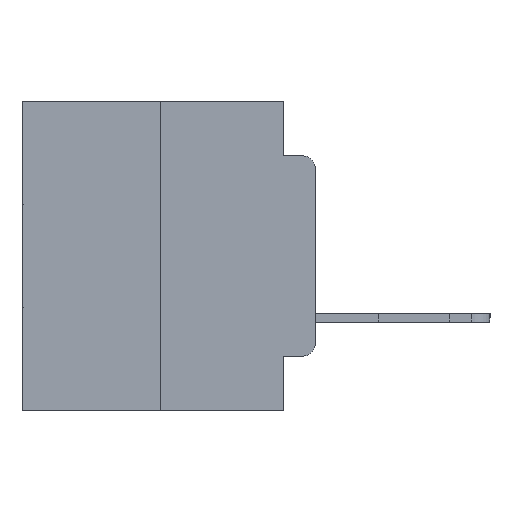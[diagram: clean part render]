
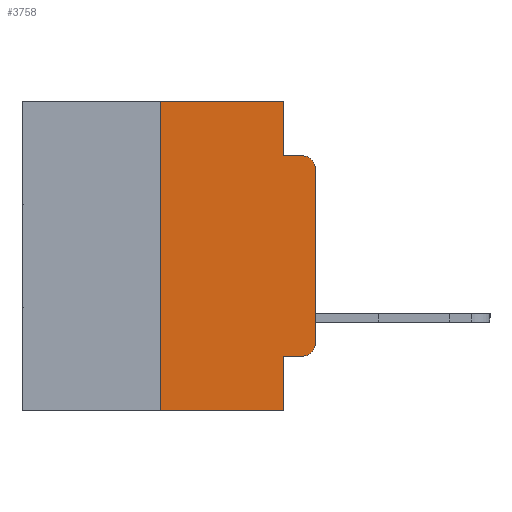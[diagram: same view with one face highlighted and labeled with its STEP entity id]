
A CAD part, left-side view. The second image highlights one B-rep face of the part: STEP entity #3758.
In plain terms, the highlighted planar face has unit normal (-1, 0, 0).
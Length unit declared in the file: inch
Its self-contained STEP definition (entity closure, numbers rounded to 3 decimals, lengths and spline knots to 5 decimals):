
#509 = VERTEX_POINT ( 'NONE', #731 ) ;
#619 = EDGE_CURVE ( 'NONE', #2781, #13525, #25787, .T. ) ;
#653 = ORIENTED_EDGE ( 'NONE', *, *, #619, .T. ) ;
#731 = CARTESIAN_POINT ( 'NONE',  ( 0., 0.25, -0.5 ) ) ;
#1536 = CARTESIAN_POINT ( 'NONE',  ( 0., 0.02, -0.4115 ) ) ;
#1886 = CARTESIAN_POINT ( 'NONE',  ( 0., 0.051, -0.0885 ) ) ;
#1912 = VECTOR ( 'NONE', #22514, 39.37008 ) ;
#2169 = ORIENTED_EDGE ( 'NONE', *, *, #4892, .T. ) ;
#2703 = EDGE_CURVE ( 'NONE', #5322, #26396, #15294, .T. ) ;
#2781 = VERTEX_POINT ( 'NONE', #17299 ) ;
#3119 = CARTESIAN_POINT ( 'NONE',  ( 0., 0.051, -0.5 ) ) ;
#3184 = CARTESIAN_POINT ( 'NONE',  ( 0., 0.25, 0. ) ) ;
#3740 = VERTEX_POINT ( 'NONE', #11287 ) ;
#3758 = ADVANCED_FACE ( 'NONE', ( #14607 ), #15090, .F. ) ;
#3760 = VECTOR ( 'NONE', #12633, 39.37008 ) ;
#4326 = ORIENTED_EDGE ( 'NONE', *, *, #18955, .F. ) ;
#4496 = DIRECTION ( 'NONE',  ( 0., -1., 0. ) ) ;
#4892 = EDGE_CURVE ( 'NONE', #13525, #3740, #17182, .T. ) ;
#5014 = ORIENTED_EDGE ( 'NONE', *, *, #11476, .T. ) ;
#5322 = VERTEX_POINT ( 'NONE', #23242 ) ;
#5421 = DIRECTION ( 'NONE',  ( 0., 0., 1. ) ) ;
#5715 = VERTEX_POINT ( 'NONE', #3119 ) ;
#7030 = ORIENTED_EDGE ( 'NONE', *, *, #26593, .T. ) ;
#7948 = CARTESIAN_POINT ( 'NONE',  ( 0., 0.473, 0. ) ) ;
#8159 = DIRECTION ( 'NONE',  ( 0., 0., -1. ) ) ;
#8310 = DIRECTION ( 'NONE',  ( 1., 0., 0. ) ) ;
#8346 = EDGE_LOOP ( 'NONE', ( #653, #2169, #19217, #15012, #25735, #4326, #5014, #10703, #22994, #7030 ) ) ;
#8348 = VERTEX_POINT ( 'NONE', #19682 ) ;
#8958 = DIRECTION ( 'NONE',  ( 0., 0., 1. ) ) ;
#9043 = DIRECTION ( 'NONE',  ( 0., -1., 0. ) ) ;
#9094 = CARTESIAN_POINT ( 'NONE',  ( 0., 0.02, -0.3915 ) ) ;
#9879 = CARTESIAN_POINT ( 'NONE',  ( 0., 0.02, -0.1085 ) ) ;
#10219 = VECTOR ( 'NONE', #9043, 39.37008 ) ;
#10496 = CARTESIAN_POINT ( 'NONE',  ( 0., 0.051, 0. ) ) ;
#10703 = ORIENTED_EDGE ( 'NONE', *, *, #16935, .F. ) ;
#11239 = DIRECTION ( 'NONE',  ( 0., 0., -1. ) ) ;
#11287 = CARTESIAN_POINT ( 'NONE',  ( 0., 0.02, -0.0885 ) ) ;
#11476 = EDGE_CURVE ( 'NONE', #509, #5715, #15886, .T. ) ;
#11786 = VECTOR ( 'NONE', #4496, 39.37008 ) ;
#11884 = CARTESIAN_POINT ( 'NONE',  ( 0., 0.051, 0. ) ) ;
#12022 = DIRECTION ( 'NONE',  ( 0., 0., -1. ) ) ;
#12633 = DIRECTION ( 'NONE',  ( 0., 0., -1. ) ) ;
#13525 = VERTEX_POINT ( 'NONE', #19213 ) ;
#14157 = LINE ( 'NONE', #14250, #23730 ) ;
#14250 = CARTESIAN_POINT ( 'NONE',  ( 0., 0.051, -0.4115 ) ) ;
#14607 = FACE_OUTER_BOUND ( 'NONE', #8346, .T. ) ;
#15012 = ORIENTED_EDGE ( 'NONE', *, *, #2703, .F. ) ;
#15090 = PLANE ( 'NONE',  #27364 ) ;
#15294 = LINE ( 'NONE', #11884, #25367 ) ;
#15638 = LINE ( 'NONE', #3184, #25050 ) ;
#15886 = LINE ( 'NONE', #23430, #10219 ) ;
#16935 = EDGE_CURVE ( 'NONE', #21772, #5715, #20590, .T. ) ;
#17063 = CARTESIAN_POINT ( 'NONE',  ( 0., 0.473, 0. ) ) ;
#17182 = CIRCLE ( 'NONE', #25048, 0.02 ) ;
#17299 = CARTESIAN_POINT ( 'NONE',  ( 0., 0., -0.3915 ) ) ;
#17381 = LINE ( 'NONE', #19032, #11786 ) ;
#17735 = CARTESIAN_POINT ( 'NONE',  ( 0., 0.051, -0.4115 ) ) ;
#18423 = CARTESIAN_POINT ( 'NONE',  ( 0., 0., 0. ) ) ;
#18464 = AXIS2_PLACEMENT_3D ( 'NONE', #9094, #23568, #11239 ) ;
#18955 = EDGE_CURVE ( 'NONE', #509, #8348, #15638, .T. ) ;
#19032 = CARTESIAN_POINT ( 'NONE',  ( 0., 0.051, -0.0885 ) ) ;
#19213 = CARTESIAN_POINT ( 'NONE',  ( 0., 0., -0.1085 ) ) ;
#19217 = ORIENTED_EDGE ( 'NONE', *, *, #26492, .F. ) ;
#19682 = CARTESIAN_POINT ( 'NONE',  ( 0., 0.25, 0. ) ) ;
#20513 = VECTOR ( 'NONE', #8958, 39.37008 ) ;
#20590 = LINE ( 'NONE', #10496, #3760 ) ;
#21488 = CIRCLE ( 'NONE', #18464, 0.02 ) ;
#21772 = VERTEX_POINT ( 'NONE', #17735 ) ;
#22514 = DIRECTION ( 'NONE',  ( 0., -1., 0. ) ) ;
#22994 = ORIENTED_EDGE ( 'NONE', *, *, #25116, .T. ) ;
#23206 = DIRECTION ( 'NONE',  ( 0., 0., -1. ) ) ;
#23242 = CARTESIAN_POINT ( 'NONE',  ( 0., 0.051, 0. ) ) ;
#23430 = CARTESIAN_POINT ( 'NONE',  ( 0., 0.473, -0.5 ) ) ;
#23568 = DIRECTION ( 'NONE',  ( -1., 0., 0. ) ) ;
#23692 = LINE ( 'NONE', #7948, #1912 ) ;
#23730 = VECTOR ( 'NONE', #26368, 39.37008 ) ;
#24265 = DIRECTION ( 'NONE',  ( -1., 0., 0. ) ) ;
#25048 = AXIS2_PLACEMENT_3D ( 'NONE', #9879, #24265, #12022 ) ;
#25050 = VECTOR ( 'NONE', #5421, 39.37008 ) ;
#25116 = EDGE_CURVE ( 'NONE', #21772, #25221, #14157, .T. ) ;
#25221 = VERTEX_POINT ( 'NONE', #1536 ) ;
#25367 = VECTOR ( 'NONE', #23206, 39.37008 ) ;
#25735 = ORIENTED_EDGE ( 'NONE', *, *, #26988, .F. ) ;
#25787 = LINE ( 'NONE', #18423, #20513 ) ;
#26368 = DIRECTION ( 'NONE',  ( 0., -1., 0. ) ) ;
#26396 = VERTEX_POINT ( 'NONE', #1886 ) ;
#26492 = EDGE_CURVE ( 'NONE', #26396, #3740, #17381, .T. ) ;
#26593 = EDGE_CURVE ( 'NONE', #25221, #2781, #21488, .T. ) ;
#26988 = EDGE_CURVE ( 'NONE', #8348, #5322, #23692, .T. ) ;
#27364 = AXIS2_PLACEMENT_3D ( 'NONE', #17063, #8310, #8159 ) ;
